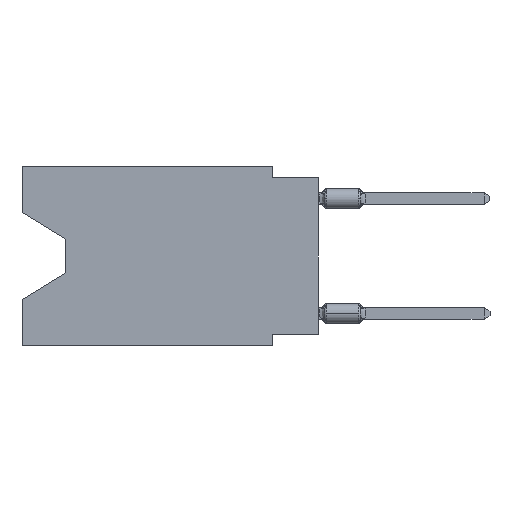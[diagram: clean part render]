
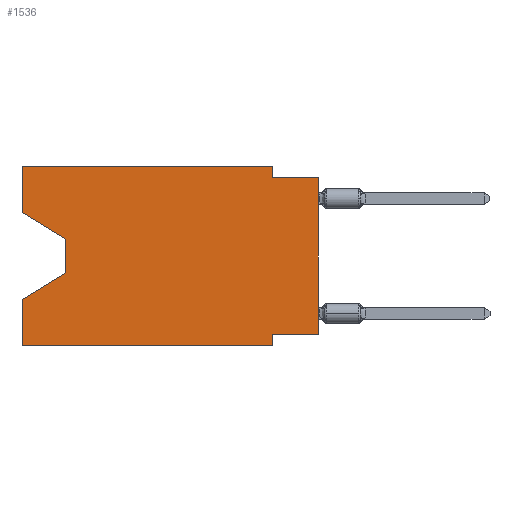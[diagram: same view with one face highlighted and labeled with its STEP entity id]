
A CAD part, left-side view. The second image highlights one B-rep face of the part: STEP entity #1536.
In plain terms, the highlighted planar face has unit normal (-1, 0, 0).
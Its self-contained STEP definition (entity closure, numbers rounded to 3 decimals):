
#177 = FACE_OUTER_BOUND ( 'NONE', #14307, .T. ) ;
#473 = ORIENTED_EDGE ( 'NONE', *, *, #9204, .F. ) ;
#593 = CARTESIAN_POINT ( 'NONE',  ( 0., 13.97, -4.013 ) ) ;
#631 = CARTESIAN_POINT ( 'NONE',  ( 0., 2.54, -9.271 ) ) ;
#703 = CARTESIAN_POINT ( 'NONE',  ( 0., 13.97, -5.893 ) ) ;
#737 = LINE ( 'NONE', #7764, #14953 ) ;
#796 = VECTOR ( 'NONE', #3985, 1000. ) ;
#819 = ORIENTED_EDGE ( 'NONE', *, *, #12842, .T. ) ;
#899 = LINE ( 'NONE', #7911, #7437 ) ;
#917 = DIRECTION ( 'NONE',  ( 0., 0., -1. ) ) ;
#1254 = LINE ( 'NONE', #22010, #4326 ) ;
#1472 = EDGE_CURVE ( 'NONE', #4460, #6926, #21384, .T. ) ;
#1536 = ADVANCED_FACE ( 'NONE', ( #177 ), #8812, .F. ) ;
#1601 = DIRECTION ( 'NONE',  ( 0., 1., 0. ) ) ;
#1770 = CARTESIAN_POINT ( 'NONE',  ( 0., 0., -9.271 ) ) ;
#1964 = CARTESIAN_POINT ( 'NONE',  ( 0., 16.383, -2.546 ) ) ;
#2113 = EDGE_CURVE ( 'NONE', #11139, #21204, #11964, .T. ) ;
#2371 = VERTEX_POINT ( 'NONE', #21071 ) ;
#3016 = CARTESIAN_POINT ( 'NONE',  ( 0., 16.383, 0. ) ) ;
#3111 = CARTESIAN_POINT ( 'NONE',  ( 0., 2.54, -9.906 ) ) ;
#3324 = CARTESIAN_POINT ( 'NONE',  ( 0., 0., -9.271 ) ) ;
#3975 = ORIENTED_EDGE ( 'NONE', *, *, #2113, .F. ) ;
#3985 = DIRECTION ( 'NONE',  ( 0., 0.855, -0.519 ) ) ;
#4326 = VECTOR ( 'NONE', #4483, 1000. ) ;
#4460 = VERTEX_POINT ( 'NONE', #703 ) ;
#4483 = DIRECTION ( 'NONE',  ( 0., 0., -1. ) ) ;
#4527 = DIRECTION ( 'NONE',  ( 0., 0., 1. ) ) ;
#4768 = ORIENTED_EDGE ( 'NONE', *, *, #22063, .F. ) ;
#5417 = EDGE_CURVE ( 'NONE', #11139, #7273, #7784, .T. ) ;
#5429 = CARTESIAN_POINT ( 'NONE',  ( 0., 0., -0.635 ) ) ;
#6690 = DIRECTION ( 'NONE',  ( 0., 0., 1. ) ) ;
#6895 = DIRECTION ( 'NONE',  ( 0., -1., 0. ) ) ;
#6926 = VERTEX_POINT ( 'NONE', #10532 ) ;
#7273 = VERTEX_POINT ( 'NONE', #5429 ) ;
#7369 = VERTEX_POINT ( 'NONE', #7492 ) ;
#7437 = VECTOR ( 'NONE', #11591, 1000. ) ;
#7492 = CARTESIAN_POINT ( 'NONE',  ( 0., 16.383, 0. ) ) ;
#7703 = ORIENTED_EDGE ( 'NONE', *, *, #18211, .F. ) ;
#7764 = CARTESIAN_POINT ( 'NONE',  ( 0., 16.383, -2.546 ) ) ;
#7784 = LINE ( 'NONE', #14816, #21000 ) ;
#7872 = VECTOR ( 'NONE', #917, 1000. ) ;
#7876 = DIRECTION ( 'NONE',  ( 0., -0.855, -0.519 ) ) ;
#7911 = CARTESIAN_POINT ( 'NONE',  ( 0., 16.383, 0. ) ) ;
#8778 = VERTEX_POINT ( 'NONE', #15422 ) ;
#8812 = PLANE ( 'NONE',  #13321 ) ;
#9201 = LINE ( 'NONE', #11610, #11173 ) ;
#9204 = EDGE_CURVE ( 'NONE', #7369, #2371, #899, .T. ) ;
#9450 = VECTOR ( 'NONE', #20645, 1000. ) ;
#9650 = DIRECTION ( 'NONE',  ( 0., -1., 0. ) ) ;
#9880 = LINE ( 'NONE', #16926, #7872 ) ;
#10532 = CARTESIAN_POINT ( 'NONE',  ( 0., 16.383, -7.36 ) ) ;
#10728 = ORIENTED_EDGE ( 'NONE', *, *, #5417, .T. ) ;
#10763 = DIRECTION ( 'NONE',  ( 1., 0., 0. ) ) ;
#11139 = VERTEX_POINT ( 'NONE', #1770 ) ;
#11173 = VECTOR ( 'NONE', #9650, 1000. ) ;
#11292 = ORIENTED_EDGE ( 'NONE', *, *, #22031, .F. ) ;
#11591 = DIRECTION ( 'NONE',  ( 0., -1., 0. ) ) ;
#11610 = CARTESIAN_POINT ( 'NONE',  ( 0., 0., -0.635 ) ) ;
#11758 = LINE ( 'NONE', #17202, #9450 ) ;
#11964 = LINE ( 'NONE', #3324, #21827 ) ;
#12107 = EDGE_CURVE ( 'NONE', #17378, #18136, #20723, .T. ) ;
#12634 = ORIENTED_EDGE ( 'NONE', *, *, #13256, .T. ) ;
#12842 = EDGE_CURVE ( 'NONE', #18325, #16812, #737, .T. ) ;
#13256 = EDGE_CURVE ( 'NONE', #16812, #4460, #11758, .T. ) ;
#13321 = AXIS2_PLACEMENT_3D ( 'NONE', #14239, #10763, #17838 ) ;
#13332 = EDGE_CURVE ( 'NONE', #18325, #7369, #13731, .T. ) ;
#13731 = LINE ( 'NONE', #3016, #22729 ) ;
#14239 = CARTESIAN_POINT ( 'NONE',  ( 0., 16.383, 0. ) ) ;
#14307 = EDGE_LOOP ( 'NONE', ( #819, #12634, #21588, #7703, #18777, #22089, #3975, #10728, #11292, #4768, #473, #15496 ) ) ;
#14816 = CARTESIAN_POINT ( 'NONE',  ( 0., 0., 0. ) ) ;
#14953 = VECTOR ( 'NONE', #7876, 1000. ) ;
#15061 = CARTESIAN_POINT ( 'NONE',  ( 0., 16.383, -9.906 ) ) ;
#15422 = CARTESIAN_POINT ( 'NONE',  ( 0., 2.54, -0.635 ) ) ;
#15429 = LINE ( 'NONE', #22494, #18193 ) ;
#15496 = ORIENTED_EDGE ( 'NONE', *, *, #13332, .F. ) ;
#16812 = VERTEX_POINT ( 'NONE', #593 ) ;
#16926 = CARTESIAN_POINT ( 'NONE',  ( 0., 2.54, 0. ) ) ;
#17202 = CARTESIAN_POINT ( 'NONE',  ( 0., 13.97, -4.013 ) ) ;
#17378 = VERTEX_POINT ( 'NONE', #15061 ) ;
#17838 = DIRECTION ( 'NONE',  ( 0., 0., -1. ) ) ;
#18136 = VERTEX_POINT ( 'NONE', #3111 ) ;
#18193 = VECTOR ( 'NONE', #6690, 1000. ) ;
#18211 = EDGE_CURVE ( 'NONE', #17378, #6926, #15429, .T. ) ;
#18325 = VERTEX_POINT ( 'NONE', #1964 ) ;
#18482 = VECTOR ( 'NONE', #6895, 1000. ) ;
#18553 = EDGE_CURVE ( 'NONE', #21204, #18136, #1254, .T. ) ;
#18777 = ORIENTED_EDGE ( 'NONE', *, *, #12107, .T. ) ;
#19905 = DIRECTION ( 'NONE',  ( 0., 0., 1. ) ) ;
#20645 = DIRECTION ( 'NONE',  ( 0., 0., -1. ) ) ;
#20723 = LINE ( 'NONE', #22357, #18482 ) ;
#21000 = VECTOR ( 'NONE', #19905, 1000. ) ;
#21071 = CARTESIAN_POINT ( 'NONE',  ( 0., 2.54, 0. ) ) ;
#21148 = CARTESIAN_POINT ( 'NONE',  ( 0., 13.97, -5.893 ) ) ;
#21204 = VERTEX_POINT ( 'NONE', #631 ) ;
#21384 = LINE ( 'NONE', #21148, #796 ) ;
#21588 = ORIENTED_EDGE ( 'NONE', *, *, #1472, .T. ) ;
#21827 = VECTOR ( 'NONE', #1601, 1000. ) ;
#22010 = CARTESIAN_POINT ( 'NONE',  ( 0., 2.54, -9.906 ) ) ;
#22031 = EDGE_CURVE ( 'NONE', #8778, #7273, #9201, .T. ) ;
#22063 = EDGE_CURVE ( 'NONE', #2371, #8778, #9880, .T. ) ;
#22089 = ORIENTED_EDGE ( 'NONE', *, *, #18553, .F. ) ;
#22357 = CARTESIAN_POINT ( 'NONE',  ( 0., 16.383, -9.906 ) ) ;
#22494 = CARTESIAN_POINT ( 'NONE',  ( 0., 16.383, 0. ) ) ;
#22729 = VECTOR ( 'NONE', #4527, 1000. ) ;
